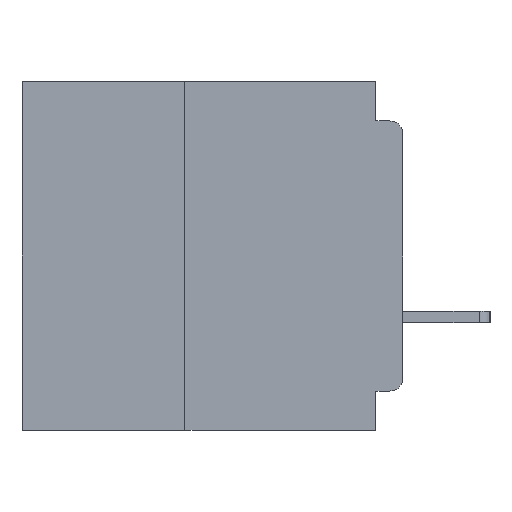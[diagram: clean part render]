
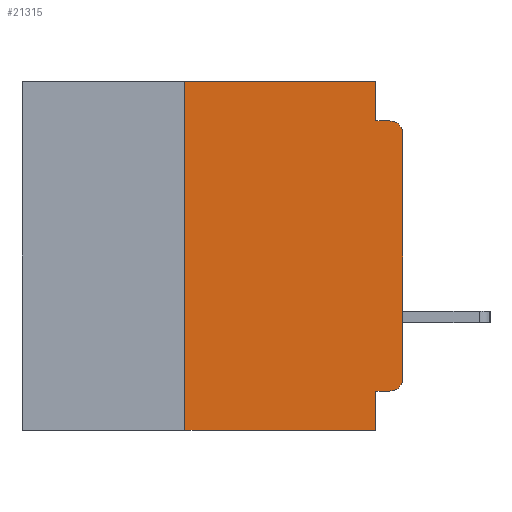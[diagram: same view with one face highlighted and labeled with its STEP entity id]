
A CAD part, left-side view. The second image highlights one B-rep face of the part: STEP entity #21315.
In plain terms, the highlighted planar face has unit normal (-1, 0, 0).
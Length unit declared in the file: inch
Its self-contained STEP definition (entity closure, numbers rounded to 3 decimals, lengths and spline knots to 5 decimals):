
#580 = VECTOR ( 'NONE', #13816, 39.37008 ) ;
#679 = ORIENTED_EDGE ( 'NONE', *, *, #20835, .F. ) ;
#897 = AXIS2_PLACEMENT_3D ( 'NONE', #10737, #34025, #14096 ) ;
#1710 = DIRECTION ( 'NONE',  ( 0., -1., 0. ) ) ;
#1827 = ORIENTED_EDGE ( 'NONE', *, *, #29669, .F. ) ;
#2445 = DIRECTION ( 'NONE',  ( 0., 0., -1. ) ) ;
#2684 = EDGE_CURVE ( 'NONE', #9766, #42918, #40487, .T. ) ;
#3331 = ORIENTED_EDGE ( 'NONE', *, *, #26915, .T. ) ;
#4941 = LINE ( 'NONE', #18411, #39347 ) ;
#6009 = CIRCLE ( 'NONE', #22580, 0.015 ) ;
#7041 = CARTESIAN_POINT ( 'NONE',  ( 0., 0.25, -0.4 ) ) ;
#7897 = DIRECTION ( 'NONE',  ( 0., 0., 1. ) ) ;
#8224 = CARTESIAN_POINT ( 'NONE',  ( 0., 0.031, 0. ) ) ;
#9038 = VECTOR ( 'NONE', #22411, 39.37008 ) ;
#9074 = CARTESIAN_POINT ( 'NONE',  ( 0., 0.437, 0. ) ) ;
#9138 = ORIENTED_EDGE ( 'NONE', *, *, #27376, .F. ) ;
#9139 = CARTESIAN_POINT ( 'NONE',  ( 0., 0., 0. ) ) ;
#9220 = ORIENTED_EDGE ( 'NONE', *, *, #38810, .F. ) ;
#9446 = CARTESIAN_POINT ( 'NONE',  ( 0., 0.031, -0.045 ) ) ;
#9549 = LINE ( 'NONE', #23751, #580 ) ;
#9711 = VECTOR ( 'NONE', #29498, 39.37008 ) ;
#9766 = VERTEX_POINT ( 'NONE', #7041 ) ;
#10063 = LINE ( 'NONE', #8224, #26718 ) ;
#10724 = CARTESIAN_POINT ( 'NONE',  ( 0., 0., -0.355 ) ) ;
#10737 = CARTESIAN_POINT ( 'NONE',  ( 0., 0.015, -0.34 ) ) ;
#11623 = DIRECTION ( 'NONE',  ( 0., 0., -1. ) ) ;
#13534 = CARTESIAN_POINT ( 'NONE',  ( 0., 0.015, -0.355 ) ) ;
#13816 = DIRECTION ( 'NONE',  ( 0., 0., -1. ) ) ;
#14096 = DIRECTION ( 'NONE',  ( 0., 0., -1. ) ) ;
#14345 = DIRECTION ( 'NONE',  ( -1., 0., 0. ) ) ;
#14605 = CARTESIAN_POINT ( 'NONE',  ( 0., 0.031, -0.355 ) ) ;
#15010 = CARTESIAN_POINT ( 'NONE',  ( 0., 0.031, -0.4 ) ) ;
#15155 = CARTESIAN_POINT ( 'NONE',  ( 0., 0.015, -0.045 ) ) ;
#16172 = EDGE_LOOP ( 'NONE', ( #3331, #40866, #679, #9138, #17032, #1827, #38385, #32657, #9220, #26948 ) ) ;
#16645 = VERTEX_POINT ( 'NONE', #28885 ) ;
#17032 = ORIENTED_EDGE ( 'NONE', *, *, #20519, .F. ) ;
#17429 = DIRECTION ( 'NONE',  ( 0., 1., 0. ) ) ;
#17922 = LINE ( 'NONE', #9139, #9038 ) ;
#18411 = CARTESIAN_POINT ( 'NONE',  ( 0., 0., -0.045 ) ) ;
#18466 = VERTEX_POINT ( 'NONE', #34915 ) ;
#19135 = PLANE ( 'NONE',  #20594 ) ;
#20400 = CIRCLE ( 'NONE', #897, 0.015 ) ;
#20519 = EDGE_CURVE ( 'NONE', #32176, #18466, #35249, .T. ) ;
#20594 = AXIS2_PLACEMENT_3D ( 'NONE', #9074, #22487, #2445 ) ;
#20835 = EDGE_CURVE ( 'NONE', #34069, #35470, #4941, .T. ) ;
#21315 = ADVANCED_FACE ( 'NONE', ( #37272 ), #19135, .F. ) ;
#22411 = DIRECTION ( 'NONE',  ( 0., 0., 1. ) ) ;
#22487 = DIRECTION ( 'NONE',  ( 1., 0., 0. ) ) ;
#22580 = AXIS2_PLACEMENT_3D ( 'NONE', #34271, #14345, #37623 ) ;
#23751 = CARTESIAN_POINT ( 'NONE',  ( 0., 0.031, -0.4 ) ) ;
#26718 = VECTOR ( 'NONE', #11623, 39.37008 ) ;
#26915 = EDGE_CURVE ( 'NONE', #16645, #29436, #17922, .T. ) ;
#26948 = ORIENTED_EDGE ( 'NONE', *, *, #29093, .T. ) ;
#27105 = VERTEX_POINT ( 'NONE', #13534 ) ;
#27140 = EDGE_CURVE ( 'NONE', #32142, #42918, #9549, .T. ) ;
#27376 = EDGE_CURVE ( 'NONE', #18466, #34069, #10063, .T. ) ;
#27876 = CARTESIAN_POINT ( 'NONE',  ( 0., 0.25, -0.4 ) ) ;
#28264 = VECTOR ( 'NONE', #7897, 39.37008 ) ;
#28885 = CARTESIAN_POINT ( 'NONE',  ( 0., 0., -0.34 ) ) ;
#29093 = EDGE_CURVE ( 'NONE', #27105, #16645, #20400, .T. ) ;
#29436 = VERTEX_POINT ( 'NONE', #36466 ) ;
#29498 = DIRECTION ( 'NONE',  ( 0., -1., 0. ) ) ;
#29669 = EDGE_CURVE ( 'NONE', #9766, #32176, #38152, .T. ) ;
#31640 = VECTOR ( 'NONE', #33492, 39.37008 ) ;
#32142 = VERTEX_POINT ( 'NONE', #14605 ) ;
#32176 = VERTEX_POINT ( 'NONE', #34676 ) ;
#32657 = ORIENTED_EDGE ( 'NONE', *, *, #27140, .F. ) ;
#33492 = DIRECTION ( 'NONE',  ( 0., -1., 0. ) ) ;
#33526 = CARTESIAN_POINT ( 'NONE',  ( 0., 0.437, -0.4 ) ) ;
#34025 = DIRECTION ( 'NONE',  ( -1., 0., 0. ) ) ;
#34069 = VERTEX_POINT ( 'NONE', #9446 ) ;
#34271 = CARTESIAN_POINT ( 'NONE',  ( 0., 0.015, -0.06 ) ) ;
#34676 = CARTESIAN_POINT ( 'NONE',  ( 0., 0.25, 0. ) ) ;
#34915 = CARTESIAN_POINT ( 'NONE',  ( 0., 0.031, 0. ) ) ;
#35249 = LINE ( 'NONE', #36034, #9711 ) ;
#35470 = VERTEX_POINT ( 'NONE', #15155 ) ;
#36034 = CARTESIAN_POINT ( 'NONE',  ( 0., 0.437, 0. ) ) ;
#36466 = CARTESIAN_POINT ( 'NONE',  ( 0., 0., -0.06 ) ) ;
#36486 = EDGE_CURVE ( 'NONE', #29436, #35470, #6009, .T. ) ;
#37272 = FACE_OUTER_BOUND ( 'NONE', #16172, .T. ) ;
#37623 = DIRECTION ( 'NONE',  ( 0., 0., -1. ) ) ;
#38136 = VECTOR ( 'NONE', #17429, 39.37008 ) ;
#38152 = LINE ( 'NONE', #27876, #28264 ) ;
#38385 = ORIENTED_EDGE ( 'NONE', *, *, #2684, .T. ) ;
#38810 = EDGE_CURVE ( 'NONE', #27105, #32142, #40208, .T. ) ;
#39347 = VECTOR ( 'NONE', #1710, 39.37008 ) ;
#40208 = LINE ( 'NONE', #10724, #38136 ) ;
#40487 = LINE ( 'NONE', #33526, #31640 ) ;
#40866 = ORIENTED_EDGE ( 'NONE', *, *, #36486, .T. ) ;
#42918 = VERTEX_POINT ( 'NONE', #15010 ) ;
